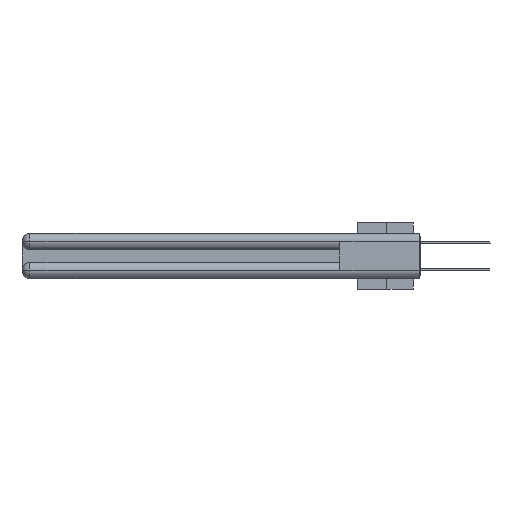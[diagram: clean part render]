
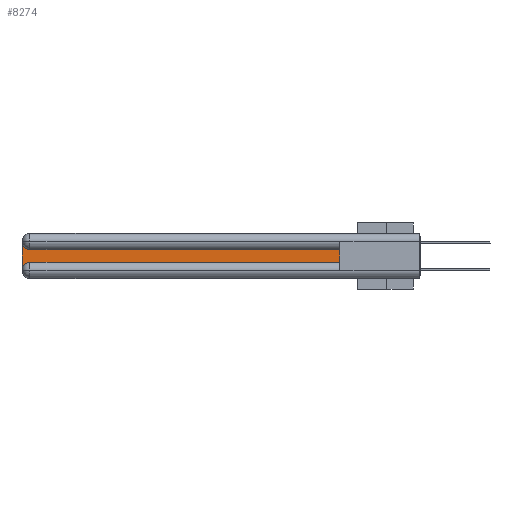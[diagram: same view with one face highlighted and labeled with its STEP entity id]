
A CAD part, left-side view. The second image highlights one B-rep face of the part: STEP entity #8274.
In plain terms, the highlighted planar face has unit normal (-1, 0, 0).
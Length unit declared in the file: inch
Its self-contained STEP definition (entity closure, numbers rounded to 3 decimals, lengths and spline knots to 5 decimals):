
#641 = CARTESIAN_POINT ( 'NONE',  ( 0.075, 2.94, -0.2175 ) ) ;
#755 = VERTEX_POINT ( 'NONE', #641 ) ;
#796 = VERTEX_POINT ( 'NONE', #18219 ) ;
#1093 = FACE_OUTER_BOUND ( 'NONE', #14683, .T. ) ;
#1647 = CARTESIAN_POINT ( 'NONE',  ( 0.075, 3., -0.1225 ) ) ;
#1898 = AXIS2_PLACEMENT_3D ( 'NONE', #1647, #4228, #29012 ) ;
#3008 = CARTESIAN_POINT ( 'NONE',  ( 0.075, 0.6, -0.1225 ) ) ;
#3478 = AXIS2_PLACEMENT_3D ( 'NONE', #14314, #11462, #9106 ) ;
#4228 = DIRECTION ( 'NONE',  ( 1., 0., 0. ) ) ;
#5129 = CARTESIAN_POINT ( 'NONE',  ( 0.075, 2.94, -0.0625 ) ) ;
#5893 = CARTESIAN_POINT ( 'NONE',  ( 0.075, 3., -0.0625 ) ) ;
#6021 = LINE ( 'NONE', #20733, #27458 ) ;
#6495 = DIRECTION ( 'NONE',  ( 0., 1., 0. ) ) ;
#6657 = VECTOR ( 'NONE', #6495, 39.37008 ) ;
#7183 = ORIENTED_EDGE ( 'NONE', *, *, #22201, .T. ) ;
#7186 = VERTEX_POINT ( 'NONE', #24324 ) ;
#7706 = DIRECTION ( 'NONE',  ( 1., 0., 0. ) ) ;
#8274 = ADVANCED_FACE ( 'NONE', ( #1093 ), #9439, .F. ) ;
#9106 = DIRECTION ( 'NONE',  ( 0., 0., -1. ) ) ;
#9439 = PLANE ( 'NONE',  #1898 ) ;
#10797 = VERTEX_POINT ( 'NONE', #3008 ) ;
#11240 = CARTESIAN_POINT ( 'NONE',  ( 0.075, 0.6, -0.2175 ) ) ;
#11462 = DIRECTION ( 'NONE',  ( 1., 0., 0. ) ) ;
#12816 = ORIENTED_EDGE ( 'NONE', *, *, #30379, .T. ) ;
#13810 = EDGE_CURVE ( 'NONE', #21772, #31911, #22853, .T. ) ;
#14176 = CARTESIAN_POINT ( 'NONE',  ( 0.075, 0.6, -0.1225 ) ) ;
#14314 = CARTESIAN_POINT ( 'NONE',  ( 0.075, 2.94, -0.2775 ) ) ;
#14625 = VECTOR ( 'NONE', #19191, 39.37008 ) ;
#14683 = EDGE_LOOP ( 'NONE', ( #27363, #7183, #18884, #20617, #26556, #12816 ) ) ;
#14764 = DIRECTION ( 'NONE',  ( 0., 0., -1. ) ) ;
#15368 = DIRECTION ( 'NONE',  ( 0., -1., 0. ) ) ;
#16552 = CARTESIAN_POINT ( 'NONE',  ( 0.075, 3., -0.2175 ) ) ;
#17932 = LINE ( 'NONE', #14176, #6657 ) ;
#18219 = CARTESIAN_POINT ( 'NONE',  ( 0.075, 2.94, -0.1225 ) ) ;
#18661 = LINE ( 'NONE', #11240, #20235 ) ;
#18842 = EDGE_CURVE ( 'NONE', #755, #7186, #6021, .T. ) ;
#18884 = ORIENTED_EDGE ( 'NONE', *, *, #13810, .T. ) ;
#19191 = DIRECTION ( 'NONE',  ( 0., 0., -1. ) ) ;
#20235 = VECTOR ( 'NONE', #26273, 39.37008 ) ;
#20617 = ORIENTED_EDGE ( 'NONE', *, *, #31363, .T. ) ;
#20733 = CARTESIAN_POINT ( 'NONE',  ( 0.075, 0.6, -0.2175 ) ) ;
#21352 = CIRCLE ( 'NONE', #3478, 0.06 ) ;
#21412 = CARTESIAN_POINT ( 'NONE',  ( 0.075, 3., -0.2775 ) ) ;
#21772 = VERTEX_POINT ( 'NONE', #5893 ) ;
#22201 = EDGE_CURVE ( 'NONE', #796, #21772, #30917, .T. ) ;
#22853 = LINE ( 'NONE', #16552, #14625 ) ;
#24282 = EDGE_CURVE ( 'NONE', #10797, #796, #17932, .T. ) ;
#24324 = CARTESIAN_POINT ( 'NONE',  ( 0.075, 0.6, -0.2175 ) ) ;
#26273 = DIRECTION ( 'NONE',  ( 0., 0., 1. ) ) ;
#26556 = ORIENTED_EDGE ( 'NONE', *, *, #18842, .T. ) ;
#27363 = ORIENTED_EDGE ( 'NONE', *, *, #24282, .T. ) ;
#27458 = VECTOR ( 'NONE', #15368, 39.37008 ) ;
#29012 = DIRECTION ( 'NONE',  ( 0., 0., -1. ) ) ;
#30379 = EDGE_CURVE ( 'NONE', #7186, #10797, #18661, .T. ) ;
#30917 = CIRCLE ( 'NONE', #31212, 0.06 ) ;
#31212 = AXIS2_PLACEMENT_3D ( 'NONE', #5129, #7706, #14764 ) ;
#31363 = EDGE_CURVE ( 'NONE', #31911, #755, #21352, .T. ) ;
#31911 = VERTEX_POINT ( 'NONE', #21412 ) ;
